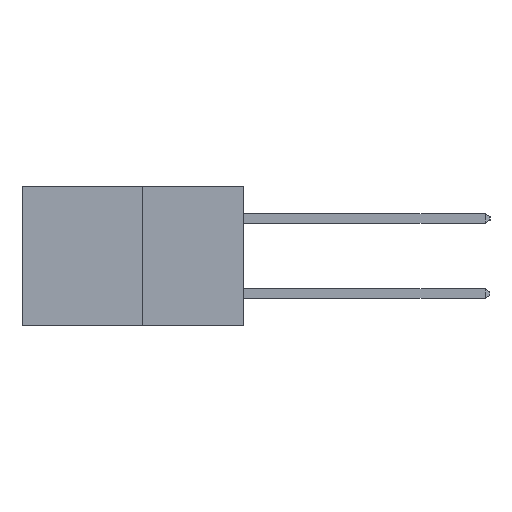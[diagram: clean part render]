
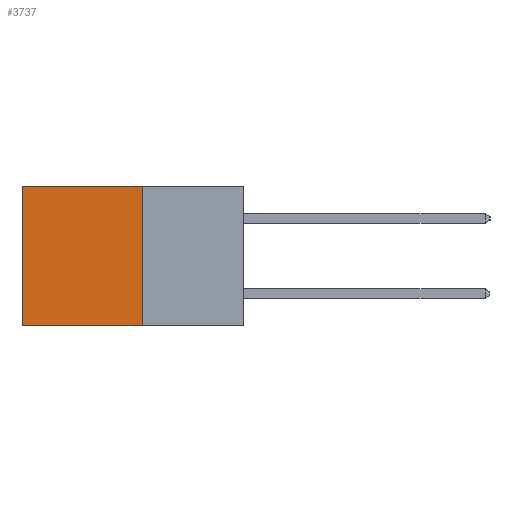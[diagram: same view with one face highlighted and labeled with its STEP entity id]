
A CAD part, left-side view. The second image highlights one B-rep face of the part: STEP entity #3737.
In plain terms, the highlighted planar face has unit normal (-1, 0, 0).
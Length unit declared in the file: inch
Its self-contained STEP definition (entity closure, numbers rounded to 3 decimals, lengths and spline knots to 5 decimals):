
#380 = VERTEX_POINT ( 'NONE', #9148 ) ;
#608 = EDGE_LOOP ( 'NONE', ( #9719, #13401, #4933, #5560 ) ) ;
#1732 = DIRECTION ( 'NONE',  ( 0., 0., -1. ) ) ;
#1872 = AXIS2_PLACEMENT_3D ( 'NONE', #7433, #12567, #10071 ) ;
#1957 = PLANE ( 'NONE',  #1872 ) ;
#2189 = EDGE_CURVE ( 'NONE', #14403, #6413, #5081, .T. ) ;
#2302 = VECTOR ( 'NONE', #6745, 39.37008 ) ;
#2402 = LINE ( 'NONE', #3813, #11172 ) ;
#3737 = ADVANCED_FACE ( 'NONE', ( #13912 ), #1957, .F. ) ;
#3813 = CARTESIAN_POINT ( 'NONE',  ( 0.277, 0.27, -0.37 ) ) ;
#3927 = EDGE_CURVE ( 'NONE', #14492, #14403, #11413, .T. ) ;
#4337 = CARTESIAN_POINT ( 'NONE',  ( 0.277, 0.27, 0. ) ) ;
#4933 = ORIENTED_EDGE ( 'NONE', *, *, #7698, .F. ) ;
#5081 = LINE ( 'NONE', #10393, #7733 ) ;
#5311 = CARTESIAN_POINT ( 'NONE',  ( 0.277, 0.59, 0. ) ) ;
#5560 = ORIENTED_EDGE ( 'NONE', *, *, #3927, .T. ) ;
#5850 = CARTESIAN_POINT ( 'NONE',  ( 0.277, 0.27, 0. ) ) ;
#6143 = DIRECTION ( 'NONE',  ( 0., 1., 0. ) ) ;
#6370 = DIRECTION ( 'NONE',  ( 0., 0., -1. ) ) ;
#6413 = VERTEX_POINT ( 'NONE', #12011 ) ;
#6745 = DIRECTION ( 'NONE',  ( 0., 1., 0. ) ) ;
#6952 = EDGE_CURVE ( 'NONE', #380, #6413, #2402, .T. ) ;
#7433 = CARTESIAN_POINT ( 'NONE',  ( 0.277, 0.27, -0.37 ) ) ;
#7698 = EDGE_CURVE ( 'NONE', #14492, #380, #12918, .T. ) ;
#7733 = VECTOR ( 'NONE', #1732, 39.37008 ) ;
#9148 = CARTESIAN_POINT ( 'NONE',  ( 0.277, 0.27, -0.37 ) ) ;
#9719 = ORIENTED_EDGE ( 'NONE', *, *, #2189, .T. ) ;
#9905 = VECTOR ( 'NONE', #6370, 39.37008 ) ;
#10071 = DIRECTION ( 'NONE',  ( 0., 0., -1. ) ) ;
#10393 = CARTESIAN_POINT ( 'NONE',  ( 0.277, 0.59, -0.37 ) ) ;
#11172 = VECTOR ( 'NONE', #6143, 39.37008 ) ;
#11413 = LINE ( 'NONE', #5850, #2302 ) ;
#12011 = CARTESIAN_POINT ( 'NONE',  ( 0.277, 0.59, -0.37 ) ) ;
#12567 = DIRECTION ( 'NONE',  ( 1., 0., 0. ) ) ;
#12918 = LINE ( 'NONE', #13017, #9905 ) ;
#13017 = CARTESIAN_POINT ( 'NONE',  ( 0.277, 0.27, -0.37 ) ) ;
#13401 = ORIENTED_EDGE ( 'NONE', *, *, #6952, .F. ) ;
#13912 = FACE_OUTER_BOUND ( 'NONE', #608, .T. ) ;
#14403 = VERTEX_POINT ( 'NONE', #5311 ) ;
#14492 = VERTEX_POINT ( 'NONE', #4337 ) ;
